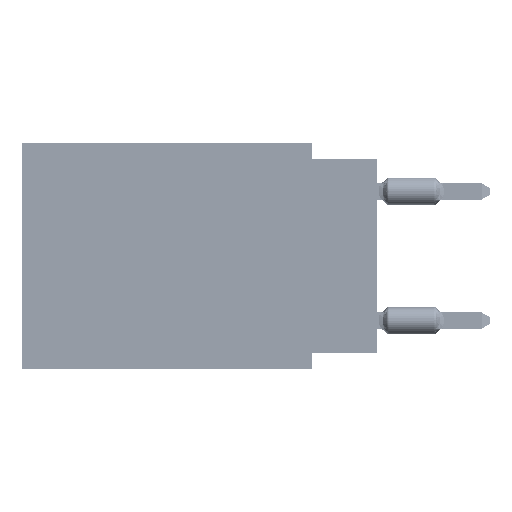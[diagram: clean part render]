
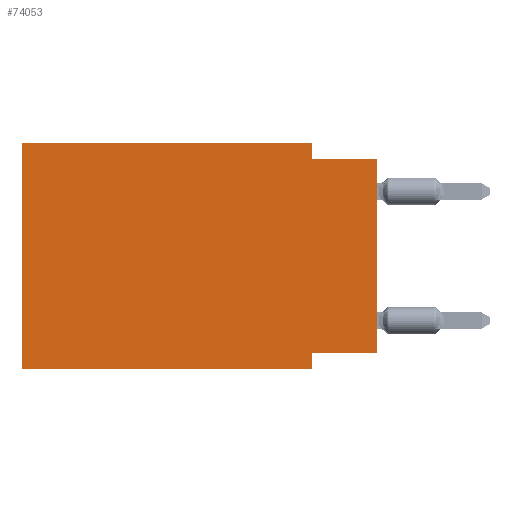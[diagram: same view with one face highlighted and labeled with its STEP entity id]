
A CAD part, left-side view. The second image highlights one B-rep face of the part: STEP entity #74053.
In plain terms, the highlighted planar face has unit normal (-1, 0, 0).
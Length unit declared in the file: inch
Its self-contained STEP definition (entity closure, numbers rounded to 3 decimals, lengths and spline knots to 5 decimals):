
#1019 = ORIENTED_EDGE ( 'NONE', *, *, #22394, .T. ) ;
#1542 = EDGE_CURVE ( 'NONE', #40199, #54287, #83679, .T. ) ;
#2736 = EDGE_CURVE ( 'NONE', #40199, #35415, #46182, .T. ) ;
#4493 = EDGE_CURVE ( 'NONE', #35415, #70785, #19598, .T. ) ;
#8064 = CARTESIAN_POINT ( 'NONE',  ( 0., 0.1, -0.325 ) ) ;
#9267 = ORIENTED_EDGE ( 'NONE', *, *, #2736, .F. ) ;
#13164 = CARTESIAN_POINT ( 'NONE',  ( 0., 0.55, 0. ) ) ;
#14697 = EDGE_CURVE ( 'NONE', #83175, #79460, #47098, .T. ) ;
#16920 = EDGE_LOOP ( 'NONE', ( #55740, #49223, #87221, #87203, #59188, #1019, #88663, #9267 ) ) ;
#16950 = EDGE_CURVE ( 'NONE', #90416, #54287, #42270, .T. ) ;
#19528 = CARTESIAN_POINT ( 'NONE',  ( 0., 0.55, -0.35 ) ) ;
#19598 = LINE ( 'NONE', #88164, #54736 ) ;
#19940 = CARTESIAN_POINT ( 'NONE',  ( 0., 0.1, -0.35 ) ) ;
#20256 = DIRECTION ( 'NONE',  ( 0., 0., -1. ) ) ;
#20351 = CARTESIAN_POINT ( 'NONE',  ( 0., 0.55, 0. ) ) ;
#20833 = DIRECTION ( 'NONE',  ( 0., -1., 0. ) ) ;
#21366 = VECTOR ( 'NONE', #20833, 39.37008 ) ;
#22394 = EDGE_CURVE ( 'NONE', #55636, #70785, #53438, .T. ) ;
#23564 = FACE_OUTER_BOUND ( 'NONE', #16920, .T. ) ;
#25288 = VECTOR ( 'NONE', #77983, 39.37008 ) ;
#28203 = EDGE_CURVE ( 'NONE', #55636, #83175, #51622, .T. ) ;
#28453 = VECTOR ( 'NONE', #76368, 39.37008 ) ;
#31018 = LINE ( 'NONE', #35070, #49682 ) ;
#33650 = DIRECTION ( 'NONE',  ( 0., -1., 0. ) ) ;
#34803 = VECTOR ( 'NONE', #33650, 39.37008 ) ;
#35070 = CARTESIAN_POINT ( 'NONE',  ( 0., 0.1, 0. ) ) ;
#35415 = VERTEX_POINT ( 'NONE', #8064 ) ;
#38294 = CARTESIAN_POINT ( 'NONE',  ( 0., 0.1, -0.025 ) ) ;
#40199 = VERTEX_POINT ( 'NONE', #85229 ) ;
#41732 = CARTESIAN_POINT ( 'NONE',  ( 0., 0.1, 0. ) ) ;
#42270 = LINE ( 'NONE', #76878, #21366 ) ;
#46182 = LINE ( 'NONE', #70952, #25288 ) ;
#47098 = LINE ( 'NONE', #69359, #28453 ) ;
#47655 = CARTESIAN_POINT ( 'NONE',  ( 0., 0., -0.025 ) ) ;
#49223 = ORIENTED_EDGE ( 'NONE', *, *, #16950, .F. ) ;
#49419 = VECTOR ( 'NONE', #67995, 39.37008 ) ;
#49624 = CARTESIAN_POINT ( 'NONE',  ( 0., 0.55, -0.35 ) ) ;
#49682 = VECTOR ( 'NONE', #83980, 39.37008 ) ;
#50397 = CARTESIAN_POINT ( 'NONE',  ( 0., 0., 0. ) ) ;
#51622 = LINE ( 'NONE', #82066, #49419 ) ;
#53354 = DIRECTION ( 'NONE',  ( 0., 0., -1. ) ) ;
#53438 = LINE ( 'NONE', #19528, #34803 ) ;
#54287 = VERTEX_POINT ( 'NONE', #47655 ) ;
#54387 = EDGE_CURVE ( 'NONE', #79460, #90416, #31018, .T. ) ;
#54736 = VECTOR ( 'NONE', #53354, 39.37008 ) ;
#55243 = PLANE ( 'NONE',  #70767 ) ;
#55636 = VERTEX_POINT ( 'NONE', #49624 ) ;
#55740 = ORIENTED_EDGE ( 'NONE', *, *, #1542, .T. ) ;
#59188 = ORIENTED_EDGE ( 'NONE', *, *, #28203, .F. ) ;
#62275 = DIRECTION ( 'NONE',  ( 1., 0., 0. ) ) ;
#64114 = DIRECTION ( 'NONE',  ( 0., 0., 1. ) ) ;
#67995 = DIRECTION ( 'NONE',  ( 0., 0., 1. ) ) ;
#69359 = CARTESIAN_POINT ( 'NONE',  ( 0., 0.55, 0. ) ) ;
#70767 = AXIS2_PLACEMENT_3D ( 'NONE', #13164, #62275, #20256 ) ;
#70785 = VERTEX_POINT ( 'NONE', #19940 ) ;
#70952 = CARTESIAN_POINT ( 'NONE',  ( 0., 0., -0.325 ) ) ;
#74053 = ADVANCED_FACE ( 'NONE', ( #23564 ), #55243, .F. ) ;
#76368 = DIRECTION ( 'NONE',  ( 0., -1., 0. ) ) ;
#76878 = CARTESIAN_POINT ( 'NONE',  ( 0., 0., -0.025 ) ) ;
#77983 = DIRECTION ( 'NONE',  ( 0., 1., 0. ) ) ;
#79460 = VERTEX_POINT ( 'NONE', #41732 ) ;
#82066 = CARTESIAN_POINT ( 'NONE',  ( 0., 0.55, 0. ) ) ;
#83175 = VERTEX_POINT ( 'NONE', #20351 ) ;
#83679 = LINE ( 'NONE', #50397, #85877 ) ;
#83980 = DIRECTION ( 'NONE',  ( 0., 0., -1. ) ) ;
#85229 = CARTESIAN_POINT ( 'NONE',  ( 0., 0., -0.325 ) ) ;
#85877 = VECTOR ( 'NONE', #64114, 39.37008 ) ;
#87203 = ORIENTED_EDGE ( 'NONE', *, *, #14697, .F. ) ;
#87221 = ORIENTED_EDGE ( 'NONE', *, *, #54387, .F. ) ;
#88164 = CARTESIAN_POINT ( 'NONE',  ( 0., 0.1, -0.35 ) ) ;
#88663 = ORIENTED_EDGE ( 'NONE', *, *, #4493, .F. ) ;
#90416 = VERTEX_POINT ( 'NONE', #38294 ) ;
